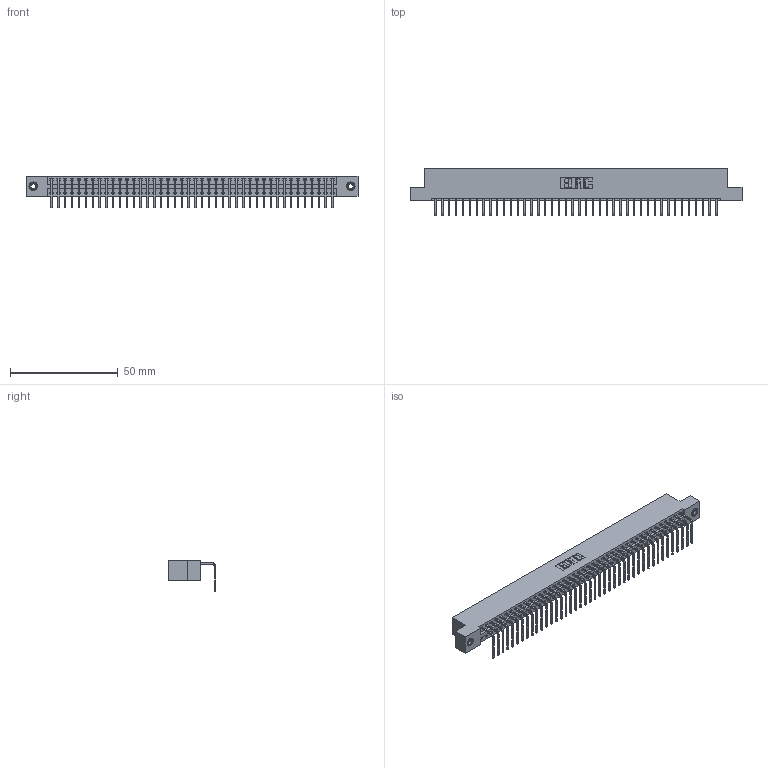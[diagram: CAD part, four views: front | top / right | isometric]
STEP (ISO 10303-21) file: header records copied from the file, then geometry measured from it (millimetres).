
FILE_DESCRIPTION (( 'STEP AP203' ), '1' );
FILE_NAME ('346-042-558-108.STEP', '2022-05-09T14:52:02', ( '' ), ( '' ), 'SwSTEP 2.0', 'SolidWorks 2020', '' );
FILE_SCHEMA (( 'CONFIG_CONTROL_DESIGN' ));
Length unit declared in the file: inch
Products named in the file (4): 345-250-001_345-250-003-102; 346-042-558-108; 346 Part_Flush Mounting Lugs - 0.156 Dia-TI; 345-292-001_558 Tail - 2
Assembly tree (45 placements, depth 2):
  346-042-558-108
    346 Part_Flush Mounting Lugs - 0.156 Dia-TI
    345-292-001_558 Tail - 2  x42
    345-250-001_345-250-003-102  x2
Bounding box: 153.92 x 22.16 x 14.73 mm (x, y, z)
Volume: 14867.4 mm3; surface area: 19438.9 mm2
Topology: 45 solids, 45 shells, 2702 faces, 8109 edges, 5342 vertices
Faces by surface type: plane 1872, cylinder 814, cone 12, torus 4
Entity records: 27336 total; most frequent: CARTESIAN_POINT 4669, ORIENTED_EDGE 4638, DIRECTION 4145, EDGE_CURVE 2319, VECTOR 1999, LINE 1999, VERTEX_POINT 1540, AXIS2_PLACEMENT_3D 1073
